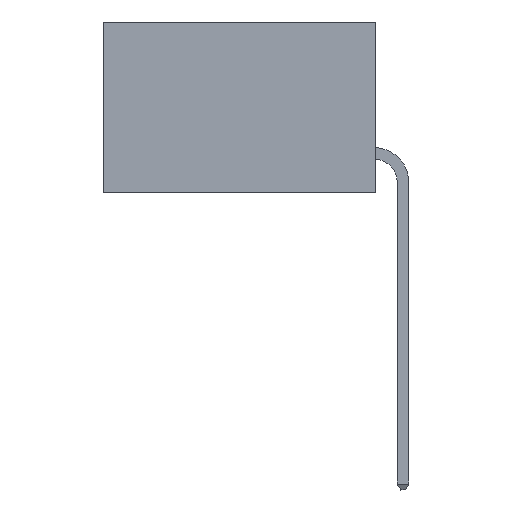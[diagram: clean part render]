
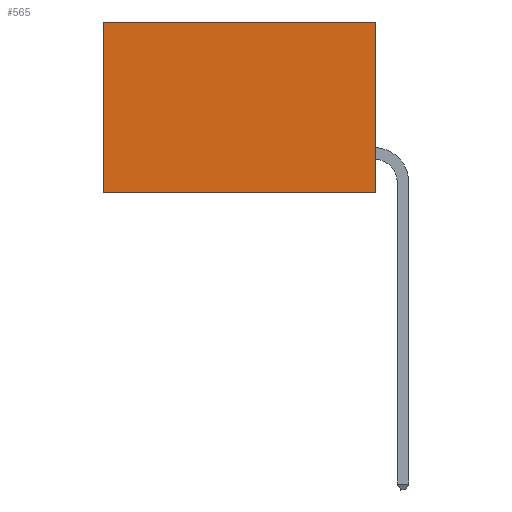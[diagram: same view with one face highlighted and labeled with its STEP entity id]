
A CAD part, left-side view. The second image highlights one B-rep face of the part: STEP entity #565.
In plain terms, the highlighted planar face has unit normal (-1, 0, 0).
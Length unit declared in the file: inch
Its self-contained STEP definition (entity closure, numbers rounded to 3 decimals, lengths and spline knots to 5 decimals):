
#33 = EDGE_CURVE ( 'NONE', #5270, #8417, #5673, .T. ) ;
#128 = LINE ( 'NONE', #4099, #5435 ) ;
#193 = EDGE_LOOP ( 'NONE', ( #6923, #7073, #562, #2583 ) ) ;
#339 = VECTOR ( 'NONE', #3710, 39.37008 ) ;
#562 = ORIENTED_EDGE ( 'NONE', *, *, #6143, .F. ) ;
#565 = ADVANCED_FACE ( 'NONE', ( #4841 ), #3860, .F. ) ;
#1218 = CARTESIAN_POINT ( 'NONE',  ( 0.277, 0.59, 0. ) ) ;
#1241 = LINE ( 'NONE', #5550, #8054 ) ;
#1429 = DIRECTION ( 'NONE',  ( 0., 1., 0. ) ) ;
#1773 = CARTESIAN_POINT ( 'NONE',  ( 0.277, 0., 0. ) ) ;
#1792 = DIRECTION ( 'NONE',  ( 1., 0., 0. ) ) ;
#2583 = ORIENTED_EDGE ( 'NONE', *, *, #33, .T. ) ;
#3710 = DIRECTION ( 'NONE',  ( 0., 1., 0. ) ) ;
#3754 = DIRECTION ( 'NONE',  ( 0., 0., -1. ) ) ;
#3829 = CARTESIAN_POINT ( 'NONE',  ( 0.277, 0., -0.37 ) ) ;
#3860 = PLANE ( 'NONE',  #6660 ) ;
#3921 = VECTOR ( 'NONE', #1429, 39.37008 ) ;
#4099 = CARTESIAN_POINT ( 'NONE',  ( 0.277, 0., -0.37 ) ) ;
#4229 = CARTESIAN_POINT ( 'NONE',  ( 0.277, 0., 0. ) ) ;
#4417 = CARTESIAN_POINT ( 'NONE',  ( 0.277, 0., -0.37 ) ) ;
#4516 = DIRECTION ( 'NONE',  ( 0., 0., -1. ) ) ;
#4841 = FACE_OUTER_BOUND ( 'NONE', #193, .T. ) ;
#5188 = CARTESIAN_POINT ( 'NONE',  ( 0.277, 0., -0.37 ) ) ;
#5270 = VERTEX_POINT ( 'NONE', #4229 ) ;
#5435 = VECTOR ( 'NONE', #3754, 39.37008 ) ;
#5488 = DIRECTION ( 'NONE',  ( 0., 0., -1. ) ) ;
#5550 = CARTESIAN_POINT ( 'NONE',  ( 0.277, 0.59, -0.37 ) ) ;
#5673 = LINE ( 'NONE', #1773, #3921 ) ;
#6041 = EDGE_CURVE ( 'NONE', #8417, #6624, #1241, .T. ) ;
#6143 = EDGE_CURVE ( 'NONE', #5270, #7099, #128, .T. ) ;
#6147 = EDGE_CURVE ( 'NONE', #7099, #6624, #7450, .T. ) ;
#6624 = VERTEX_POINT ( 'NONE', #7677 ) ;
#6660 = AXIS2_PLACEMENT_3D ( 'NONE', #4417, #1792, #4516 ) ;
#6923 = ORIENTED_EDGE ( 'NONE', *, *, #6041, .T. ) ;
#7073 = ORIENTED_EDGE ( 'NONE', *, *, #6147, .F. ) ;
#7099 = VERTEX_POINT ( 'NONE', #5188 ) ;
#7450 = LINE ( 'NONE', #3829, #339 ) ;
#7677 = CARTESIAN_POINT ( 'NONE',  ( 0.277, 0.59, -0.37 ) ) ;
#8054 = VECTOR ( 'NONE', #5488, 39.37008 ) ;
#8417 = VERTEX_POINT ( 'NONE', #1218 ) ;
